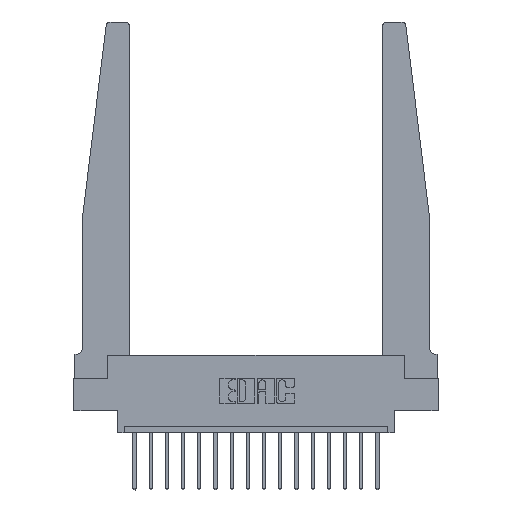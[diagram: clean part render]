
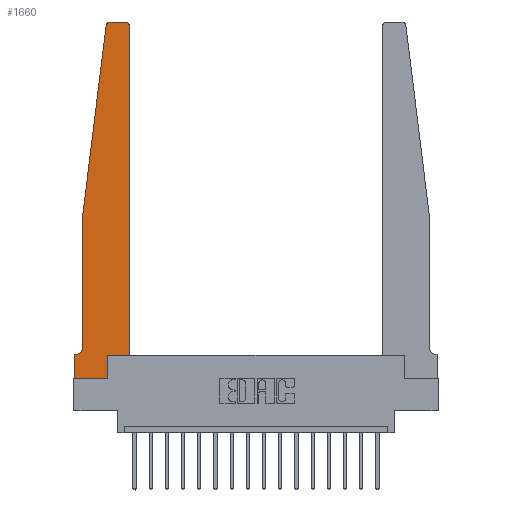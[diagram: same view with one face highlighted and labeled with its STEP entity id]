
A CAD part, top view. The second image highlights one B-rep face of the part: STEP entity #1660.
In plain terms, the highlighted planar face has unit normal (0, 0, 1).
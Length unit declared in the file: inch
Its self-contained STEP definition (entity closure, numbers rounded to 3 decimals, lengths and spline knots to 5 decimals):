
#46 = DIRECTION ( 'NONE',  ( 0., 0., 1. ) ) ;
#240 = EDGE_CURVE ( 'NONE', #18271, #9033, #8418, .T. ) ;
#295 = CARTESIAN_POINT ( 'NONE',  ( 0.25, 2.75, 0.37 ) ) ;
#356 = CIRCLE ( 'NONE', #10863, 0.03 ) ;
#361 = CARTESIAN_POINT ( 'NONE',  ( 0.015, 0.1875, 0.37 ) ) ;
#878 = VECTOR ( 'NONE', #13159, 39.37008 ) ;
#977 = VERTEX_POINT ( 'NONE', #4092 ) ;
#1210 = VERTEX_POINT ( 'NONE', #16151 ) ;
#1316 = ORIENTED_EDGE ( 'NONE', *, *, #240, .T. ) ;
#1321 = CARTESIAN_POINT ( 'NONE',  ( 0., 0.1875, 0.37 ) ) ;
#1494 = LINE ( 'NONE', #8448, #7018 ) ;
#1620 = LINE ( 'NONE', #14103, #4717 ) ;
#1660 = ADVANCED_FACE ( 'NONE', ( #15410 ), #9573, .T. ) ;
#1840 = VERTEX_POINT ( 'NONE', #15621 ) ;
#1848 = VECTOR ( 'NONE', #10638, 39.37008 ) ;
#1884 = DIRECTION ( 'NONE',  ( 1., 0., 0. ) ) ;
#1936 = EDGE_CURVE ( 'NONE', #1210, #18271, #3841, .T. ) ;
#2034 = DIRECTION ( 'NONE',  ( -0.122, -0.992, 0. ) ) ;
#2068 = CARTESIAN_POINT ( 'NONE',  ( 0.065, 1.25, 0.37 ) ) ;
#2396 = CARTESIAN_POINT ( 'NONE',  ( 0.425, 0.18, 0.37 ) ) ;
#2437 = EDGE_CURVE ( 'NONE', #17439, #8474, #16794, .T. ) ;
#2883 = DIRECTION ( 'NONE',  ( 1., 0., 0. ) ) ;
#3021 = VECTOR ( 'NONE', #8997, 39.37008 ) ;
#3083 = AXIS2_PLACEMENT_3D ( 'NONE', #5113, #16508, #17807 ) ;
#3237 = LINE ( 'NONE', #295, #3021 ) ;
#3298 = ORIENTED_EDGE ( 'NONE', *, *, #8752, .T. ) ;
#3400 = LINE ( 'NONE', #12617, #10296 ) ;
#3642 = ORIENTED_EDGE ( 'NONE', *, *, #9617, .T. ) ;
#3841 = LINE ( 'NONE', #2068, #1848 ) ;
#3870 = CARTESIAN_POINT ( 'NONE',  ( 0.015, 0.2375, 0.37 ) ) ;
#3879 = ORIENTED_EDGE ( 'NONE', *, *, #15708, .T. ) ;
#4073 = DIRECTION ( 'NONE',  ( 0., 1., 0. ) ) ;
#4092 = CARTESIAN_POINT ( 'NONE',  ( 0.24675, 2.72367, 0.37 ) ) ;
#4409 = ORIENTED_EDGE ( 'NONE', *, *, #11797, .T. ) ;
#4531 = ORIENTED_EDGE ( 'NONE', *, *, #2437, .T. ) ;
#4717 = VECTOR ( 'NONE', #13738, 39.37008 ) ;
#5113 = CARTESIAN_POINT ( 'NONE',  ( 0., 0.1875, 0.37 ) ) ;
#5488 = EDGE_CURVE ( 'NONE', #977, #1210, #11236, .T. ) ;
#5851 = ORIENTED_EDGE ( 'NONE', *, *, #1936, .T. ) ;
#6321 = ORIENTED_EDGE ( 'NONE', *, *, #7750, .T. ) ;
#6523 = DIRECTION ( 'NONE',  ( 0., 0., -1. ) ) ;
#6588 = CARTESIAN_POINT ( 'NONE',  ( 0., 0., 0.37 ) ) ;
#6822 = VECTOR ( 'NONE', #15194, 39.37008 ) ;
#6919 = VERTEX_POINT ( 'NONE', #11894 ) ;
#7018 = VECTOR ( 'NONE', #8320, 39.37008 ) ;
#7083 = CARTESIAN_POINT ( 'NONE',  ( 0.27653, 2.72, 0.37 ) ) ;
#7368 = CARTESIAN_POINT ( 'NONE',  ( 0.425, 0.18, 0.37 ) ) ;
#7442 = DIRECTION ( 'NONE',  ( 0., 0., 1. ) ) ;
#7750 = EDGE_CURVE ( 'NONE', #1840, #977, #356, .T. ) ;
#8188 = DIRECTION ( 'NONE',  ( -1., 0., 0. ) ) ;
#8320 = DIRECTION ( 'NONE',  ( -1., 0., 0. ) ) ;
#8418 = CIRCLE ( 'NONE', #12708, 0.05 ) ;
#8448 = CARTESIAN_POINT ( 'NONE',  ( 0.065, 0.1875, 0.37 ) ) ;
#8474 = VERTEX_POINT ( 'NONE', #15910 ) ;
#8752 = EDGE_CURVE ( 'NONE', #15101, #6919, #13055, .T. ) ;
#8917 = CARTESIAN_POINT ( 'NONE',  ( 0.395, 2.72, 0.37 ) ) ;
#8997 = DIRECTION ( 'NONE',  ( -1., 0., 0. ) ) ;
#9033 = VERTEX_POINT ( 'NONE', #361 ) ;
#9147 = CARTESIAN_POINT ( 'NONE',  ( 0.065, 1.25, 0.37 ) ) ;
#9466 = EDGE_LOOP ( 'NONE', ( #3879, #6321, #18007, #5851, #1316, #3642, #13289, #3298, #13286, #4409, #4531, #11736 ) ) ;
#9573 = PLANE ( 'NONE',  #3083 ) ;
#9617 = EDGE_CURVE ( 'NONE', #9033, #18297, #1494, .T. ) ;
#9725 = VECTOR ( 'NONE', #2034, 39.37008 ) ;
#10296 = VECTOR ( 'NONE', #4073, 39.37008 ) ;
#10638 = DIRECTION ( 'NONE',  ( 0., -1., 0. ) ) ;
#10863 = AXIS2_PLACEMENT_3D ( 'NONE', #7083, #46, #2883 ) ;
#11236 = LINE ( 'NONE', #9147, #9725 ) ;
#11736 = ORIENTED_EDGE ( 'NONE', *, *, #17296, .T. ) ;
#11797 = EDGE_CURVE ( 'NONE', #14382, #17439, #1620, .T. ) ;
#11894 = CARTESIAN_POINT ( 'NONE',  ( 0.2605, 0., 0.37 ) ) ;
#12617 = CARTESIAN_POINT ( 'NONE',  ( 0.2605, 0.18, 0.37 ) ) ;
#12708 = AXIS2_PLACEMENT_3D ( 'NONE', #3870, #6523, #8188 ) ;
#12777 = CARTESIAN_POINT ( 'NONE',  ( 0.065, 0.2375, 0.37 ) ) ;
#13055 = LINE ( 'NONE', #16265, #16384 ) ;
#13159 = DIRECTION ( 'NONE',  ( 0., -1., 0. ) ) ;
#13286 = ORIENTED_EDGE ( 'NONE', *, *, #17581, .T. ) ;
#13289 = ORIENTED_EDGE ( 'NONE', *, *, #14507, .T. ) ;
#13738 = DIRECTION ( 'NONE',  ( 1., 0., 0. ) ) ;
#14019 = CIRCLE ( 'NONE', #14907, 0.03 ) ;
#14103 = CARTESIAN_POINT ( 'NONE',  ( 0.425, 0.18, 0.37 ) ) ;
#14144 = CARTESIAN_POINT ( 'NONE',  ( 0.2605, 0.18, 0.37 ) ) ;
#14382 = VERTEX_POINT ( 'NONE', #14144 ) ;
#14507 = EDGE_CURVE ( 'NONE', #18297, #15101, #18134, .T. ) ;
#14907 = AXIS2_PLACEMENT_3D ( 'NONE', #8917, #7442, #1884 ) ;
#15101 = VERTEX_POINT ( 'NONE', #6588 ) ;
#15194 = DIRECTION ( 'NONE',  ( 0., 1., 0. ) ) ;
#15410 = FACE_OUTER_BOUND ( 'NONE', #9466, .T. ) ;
#15621 = CARTESIAN_POINT ( 'NONE',  ( 0.27653, 2.75, 0.37 ) ) ;
#15708 = EDGE_CURVE ( 'NONE', #16516, #1840, #3237, .T. ) ;
#15709 = CARTESIAN_POINT ( 'NONE',  ( 0.395, 2.75, 0.37 ) ) ;
#15910 = CARTESIAN_POINT ( 'NONE',  ( 0.425, 2.72, 0.37 ) ) ;
#15932 = CARTESIAN_POINT ( 'NONE',  ( 0., 0., 0.37 ) ) ;
#16151 = CARTESIAN_POINT ( 'NONE',  ( 0.065, 1.25, 0.37 ) ) ;
#16265 = CARTESIAN_POINT ( 'NONE',  ( 0., 0., 0.37 ) ) ;
#16330 = DIRECTION ( 'NONE',  ( 1., 0., 0. ) ) ;
#16384 = VECTOR ( 'NONE', #16330, 39.37008 ) ;
#16508 = DIRECTION ( 'NONE',  ( 0., 0., 1. ) ) ;
#16516 = VERTEX_POINT ( 'NONE', #15709 ) ;
#16794 = LINE ( 'NONE', #2396, #6822 ) ;
#17296 = EDGE_CURVE ( 'NONE', #8474, #16516, #14019, .T. ) ;
#17439 = VERTEX_POINT ( 'NONE', #7368 ) ;
#17581 = EDGE_CURVE ( 'NONE', #6919, #14382, #3400, .T. ) ;
#17807 = DIRECTION ( 'NONE',  ( 1., 0., 0. ) ) ;
#18007 = ORIENTED_EDGE ( 'NONE', *, *, #5488, .T. ) ;
#18134 = LINE ( 'NONE', #15932, #878 ) ;
#18271 = VERTEX_POINT ( 'NONE', #12777 ) ;
#18297 = VERTEX_POINT ( 'NONE', #1321 ) ;
